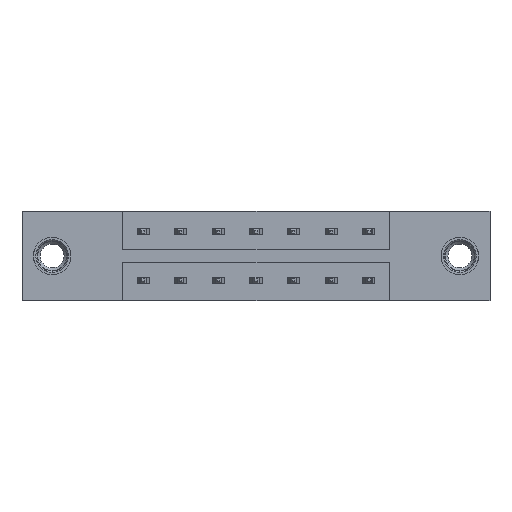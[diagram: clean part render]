
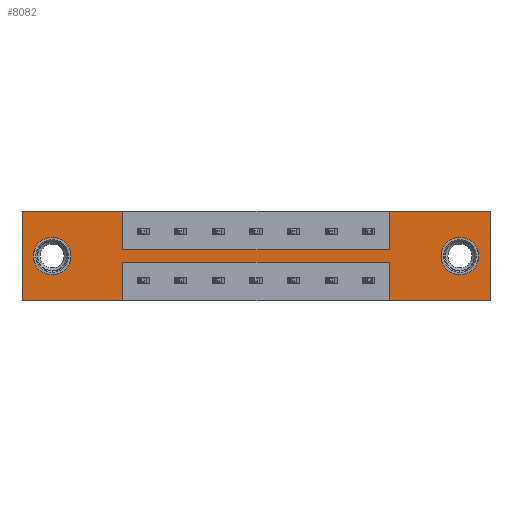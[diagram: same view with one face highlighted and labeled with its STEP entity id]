
A CAD part, front view. The second image highlights one B-rep face of the part: STEP entity #8082.
In plain terms, the highlighted planar face has unit normal (0, -1, 0).
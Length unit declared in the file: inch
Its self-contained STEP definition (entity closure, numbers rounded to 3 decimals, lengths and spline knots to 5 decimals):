
#18 = DIRECTION ( 'NONE',  ( 0., 0., 1. ) ) ;
#169 = DIRECTION ( 'NONE',  ( 0., 0., 1. ) ) ;
#208 = CARTESIAN_POINT ( 'NONE',  ( 1.5225, 0., -0.2115 ) ) ;
#271 = CIRCLE ( 'NONE', #2927, 0.078 ) ;
#475 = FACE_OUTER_BOUND ( 'NONE', #2057, .T. ) ;
#524 = LINE ( 'NONE', #574, #4256 ) ;
#528 = CARTESIAN_POINT ( 'NONE',  ( 1.5225, 0., -0.2115 ) ) ;
#531 = DIRECTION ( 'NONE',  ( 0., 1., 0. ) ) ;
#540 = ORIENTED_EDGE ( 'NONE', *, *, #5912, .F. ) ;
#568 = CARTESIAN_POINT ( 'NONE',  ( 1.815, 0., -0.185 ) ) ;
#574 = CARTESIAN_POINT ( 'NONE',  ( 1.5225, 0., -0.1585 ) ) ;
#577 = VERTEX_POINT ( 'NONE', #902 ) ;
#618 = PLANE ( 'NONE',  #8110 ) ;
#717 = CARTESIAN_POINT ( 'NONE',  ( 0.4175, 0., -0.2115 ) ) ;
#784 = VERTEX_POINT ( 'NONE', #9886 ) ;
#855 = CARTESIAN_POINT ( 'NONE',  ( 0.4175, 0., -0.2115 ) ) ;
#902 = CARTESIAN_POINT ( 'NONE',  ( 0., 0., -0.37 ) ) ;
#926 = DIRECTION ( 'NONE',  ( 0., 0., -1. ) ) ;
#1190 = CARTESIAN_POINT ( 'NONE',  ( 0., 0., -0.37 ) ) ;
#1216 = ORIENTED_EDGE ( 'NONE', *, *, #4072, .F. ) ;
#1303 = LINE ( 'NONE', #528, #10208 ) ;
#1307 = CARTESIAN_POINT ( 'NONE',  ( 0.125, 0., -0.185 ) ) ;
#1320 = DIRECTION ( 'NONE',  ( 1., 0., 0. ) ) ;
#1331 = EDGE_CURVE ( 'NONE', #5292, #6510, #524, .T. ) ;
#1352 = AXIS2_PLACEMENT_3D ( 'NONE', #9560, #1771, #169 ) ;
#1387 = EDGE_CURVE ( 'NONE', #4093, #2327, #5471, .T. ) ;
#1396 = CARTESIAN_POINT ( 'NONE',  ( 1.815, 0., -0.263 ) ) ;
#1414 = AXIS2_PLACEMENT_3D ( 'NONE', #4264, #8841, #926 ) ;
#1426 = VERTEX_POINT ( 'NONE', #1396 ) ;
#1552 = VECTOR ( 'NONE', #7143, 39.37008 ) ;
#1771 = DIRECTION ( 'NONE',  ( 0., 1., 0. ) ) ;
#1810 = LINE ( 'NONE', #4056, #5266 ) ;
#1853 = CARTESIAN_POINT ( 'NONE',  ( 0.4175, 0., -0.1585 ) ) ;
#1946 = CARTESIAN_POINT ( 'NONE',  ( 0.4175, 0., -0.1585 ) ) ;
#2012 = VERTEX_POINT ( 'NONE', #7491 ) ;
#2057 = EDGE_LOOP ( 'NONE', ( #6014, #6855, #6894, #10205, #2803, #540, #1216, #7631, #3615, #7215, #7256, #9253 ) ) ;
#2327 = VERTEX_POINT ( 'NONE', #6218 ) ;
#2436 = CARTESIAN_POINT ( 'NONE',  ( 1.5225, 0., -0.1585 ) ) ;
#2505 = CARTESIAN_POINT ( 'NONE',  ( 0.125, 0., -0.107 ) ) ;
#2580 = CARTESIAN_POINT ( 'NONE',  ( 0., 0., -0.37 ) ) ;
#2617 = EDGE_CURVE ( 'NONE', #8478, #8056, #7867, .T. ) ;
#2646 = CARTESIAN_POINT ( 'NONE',  ( 1.94, 0., -0.37 ) ) ;
#2699 = EDGE_CURVE ( 'NONE', #5010, #2012, #6556, .T. ) ;
#2803 = ORIENTED_EDGE ( 'NONE', *, *, #1331, .F. ) ;
#2869 = CARTESIAN_POINT ( 'NONE',  ( 0., 0., -0.37 ) ) ;
#2885 = DIRECTION ( 'NONE',  ( 1., 0., 0. ) ) ;
#2927 = AXIS2_PLACEMENT_3D ( 'NONE', #1307, #531, #8790 ) ;
#2931 = ORIENTED_EDGE ( 'NONE', *, *, #2699, .T. ) ;
#3085 = AXIS2_PLACEMENT_3D ( 'NONE', #568, #7554, #8375 ) ;
#3086 = VECTOR ( 'NONE', #9403, 39.37008 ) ;
#3198 = VERTEX_POINT ( 'NONE', #7902 ) ;
#3234 = CARTESIAN_POINT ( 'NONE',  ( 0., 0., 0. ) ) ;
#3275 = DIRECTION ( 'NONE',  ( 0., 0., -1. ) ) ;
#3520 = DIRECTION ( 'NONE',  ( -1., 0., 0. ) ) ;
#3615 = ORIENTED_EDGE ( 'NONE', *, *, #9150, .F. ) ;
#3635 = ORIENTED_EDGE ( 'NONE', *, *, #6596, .T. ) ;
#3704 = DIRECTION ( 'NONE',  ( 0., 0., 1. ) ) ;
#3814 = DIRECTION ( 'NONE',  ( 0., 0., 1. ) ) ;
#3818 = VERTEX_POINT ( 'NONE', #6825 ) ;
#4056 = CARTESIAN_POINT ( 'NONE',  ( 1.94, 0., 0. ) ) ;
#4072 = EDGE_CURVE ( 'NONE', #3198, #4828, #9754, .T. ) ;
#4093 = VERTEX_POINT ( 'NONE', #2646 ) ;
#4164 = DIRECTION ( 'NONE',  ( 0., 0., -1. ) ) ;
#4197 = DIRECTION ( 'NONE',  ( 0., 0., -1. ) ) ;
#4253 = VECTOR ( 'NONE', #2885, 39.37008 ) ;
#4256 = VECTOR ( 'NONE', #3704, 39.37008 ) ;
#4264 = CARTESIAN_POINT ( 'NONE',  ( 1.815, 0., -0.185 ) ) ;
#4424 = CIRCLE ( 'NONE', #1414, 0.078 ) ;
#4675 = EDGE_CURVE ( 'NONE', #2327, #8478, #1303, .T. ) ;
#4828 = VERTEX_POINT ( 'NONE', #7870 ) ;
#4940 = VECTOR ( 'NONE', #4197, 39.37008 ) ;
#5010 = VERTEX_POINT ( 'NONE', #2505 ) ;
#5161 = EDGE_CURVE ( 'NONE', #5678, #1426, #5754, .T. ) ;
#5174 = CARTESIAN_POINT ( 'NONE',  ( 0.4175, 0., -0.2115 ) ) ;
#5266 = VECTOR ( 'NONE', #3275, 39.37008 ) ;
#5292 = VERTEX_POINT ( 'NONE', #2436 ) ;
#5364 = EDGE_CURVE ( 'NONE', #3818, #4093, #1810, .T. ) ;
#5411 = VECTOR ( 'NONE', #4164, 39.37008 ) ;
#5468 = EDGE_CURVE ( 'NONE', #784, #3198, #5774, .T. ) ;
#5471 = LINE ( 'NONE', #2869, #3086 ) ;
#5678 = VERTEX_POINT ( 'NONE', #8519 ) ;
#5754 = CIRCLE ( 'NONE', #3085, 0.078 ) ;
#5774 = LINE ( 'NONE', #6605, #6257 ) ;
#5794 = EDGE_CURVE ( 'NONE', #8056, #9054, #6592, .T. ) ;
#5828 = DIRECTION ( 'NONE',  ( 1., 0., 0. ) ) ;
#5880 = VECTOR ( 'NONE', #1320, 39.37008 ) ;
#5912 = EDGE_CURVE ( 'NONE', #4828, #5292, #5913, .T. ) ;
#5913 = LINE ( 'NONE', #1946, #4253 ) ;
#6014 = ORIENTED_EDGE ( 'NONE', *, *, #4675, .F. ) ;
#6207 = VECTOR ( 'NONE', #3520, 39.37008 ) ;
#6218 = CARTESIAN_POINT ( 'NONE',  ( 1.5225, 0., -0.37 ) ) ;
#6257 = VECTOR ( 'NONE', #5828, 39.37008 ) ;
#6469 = EDGE_CURVE ( 'NONE', #2012, #5010, #271, .T. ) ;
#6510 = VERTEX_POINT ( 'NONE', #7909 ) ;
#6556 = CIRCLE ( 'NONE', #1352, 0.078 ) ;
#6592 = LINE ( 'NONE', #855, #4940 ) ;
#6596 = EDGE_CURVE ( 'NONE', #1426, #5678, #4424, .T. ) ;
#6605 = CARTESIAN_POINT ( 'NONE',  ( 0., 0., 0. ) ) ;
#6735 = ORIENTED_EDGE ( 'NONE', *, *, #6469, .T. ) ;
#6746 = CARTESIAN_POINT ( 'NONE',  ( 0., 0., 0. ) ) ;
#6776 = DIRECTION ( 'NONE',  ( 0., -1., 0. ) ) ;
#6825 = CARTESIAN_POINT ( 'NONE',  ( 1.94, 0., 0. ) ) ;
#6827 = FACE_BOUND ( 'NONE', #7727, .T. ) ;
#6855 = ORIENTED_EDGE ( 'NONE', *, *, #1387, .F. ) ;
#6894 = ORIENTED_EDGE ( 'NONE', *, *, #5364, .F. ) ;
#6985 = DIRECTION ( 'NONE',  ( 0., 0., -1. ) ) ;
#7143 = DIRECTION ( 'NONE',  ( -1., 0., 0. ) ) ;
#7215 = ORIENTED_EDGE ( 'NONE', *, *, #8961, .F. ) ;
#7256 = ORIENTED_EDGE ( 'NONE', *, *, #5794, .F. ) ;
#7491 = CARTESIAN_POINT ( 'NONE',  ( 0.125, 0., -0.263 ) ) ;
#7554 = DIRECTION ( 'NONE',  ( 0., 1., 0. ) ) ;
#7631 = ORIENTED_EDGE ( 'NONE', *, *, #5468, .F. ) ;
#7641 = LINE ( 'NONE', #6746, #5880 ) ;
#7722 = VECTOR ( 'NONE', #18, 39.37008 ) ;
#7727 = EDGE_LOOP ( 'NONE', ( #2931, #6735 ) ) ;
#7867 = LINE ( 'NONE', #717, #1552 ) ;
#7870 = CARTESIAN_POINT ( 'NONE',  ( 0.4175, 0., -0.1585 ) ) ;
#7890 = ORIENTED_EDGE ( 'NONE', *, *, #5161, .T. ) ;
#7902 = CARTESIAN_POINT ( 'NONE',  ( 0.4175, 0., 0. ) ) ;
#7909 = CARTESIAN_POINT ( 'NONE',  ( 1.5225, 0., 0. ) ) ;
#8056 = VERTEX_POINT ( 'NONE', #5174 ) ;
#8082 = ADVANCED_FACE ( 'NONE', ( #8334, #6827, #475 ), #618, .T. ) ;
#8110 = AXIS2_PLACEMENT_3D ( 'NONE', #1190, #6776, #6985 ) ;
#8334 = FACE_BOUND ( 'NONE', #9182, .T. ) ;
#8375 = DIRECTION ( 'NONE',  ( 0., 0., -1. ) ) ;
#8478 = VERTEX_POINT ( 'NONE', #208 ) ;
#8519 = CARTESIAN_POINT ( 'NONE',  ( 1.815, 0., -0.107 ) ) ;
#8790 = DIRECTION ( 'NONE',  ( 0., 0., 1. ) ) ;
#8841 = DIRECTION ( 'NONE',  ( 0., 1., 0. ) ) ;
#8961 = EDGE_CURVE ( 'NONE', #9054, #577, #9687, .T. ) ;
#9049 = EDGE_CURVE ( 'NONE', #6510, #3818, #7641, .T. ) ;
#9054 = VERTEX_POINT ( 'NONE', #9412 ) ;
#9150 = EDGE_CURVE ( 'NONE', #577, #784, #9566, .T. ) ;
#9182 = EDGE_LOOP ( 'NONE', ( #7890, #3635 ) ) ;
#9253 = ORIENTED_EDGE ( 'NONE', *, *, #2617, .F. ) ;
#9403 = DIRECTION ( 'NONE',  ( -1., 0., 0. ) ) ;
#9412 = CARTESIAN_POINT ( 'NONE',  ( 0.4175, 0., -0.37 ) ) ;
#9560 = CARTESIAN_POINT ( 'NONE',  ( 0.125, 0., -0.185 ) ) ;
#9566 = LINE ( 'NONE', #3234, #7722 ) ;
#9687 = LINE ( 'NONE', #2580, #6207 ) ;
#9754 = LINE ( 'NONE', #1853, #5411 ) ;
#9886 = CARTESIAN_POINT ( 'NONE',  ( 0., 0., 0. ) ) ;
#10205 = ORIENTED_EDGE ( 'NONE', *, *, #9049, .F. ) ;
#10208 = VECTOR ( 'NONE', #3814, 39.37008 ) ;
